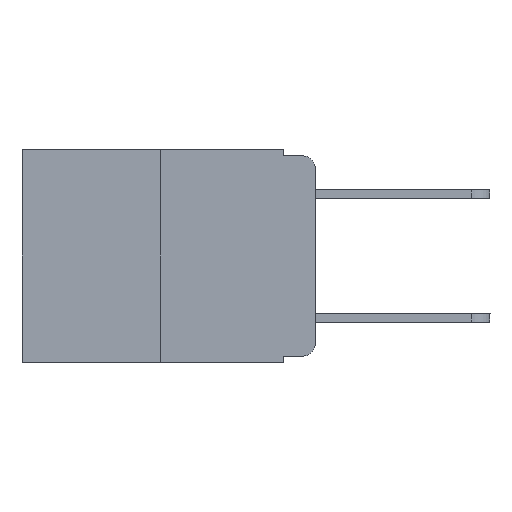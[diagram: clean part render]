
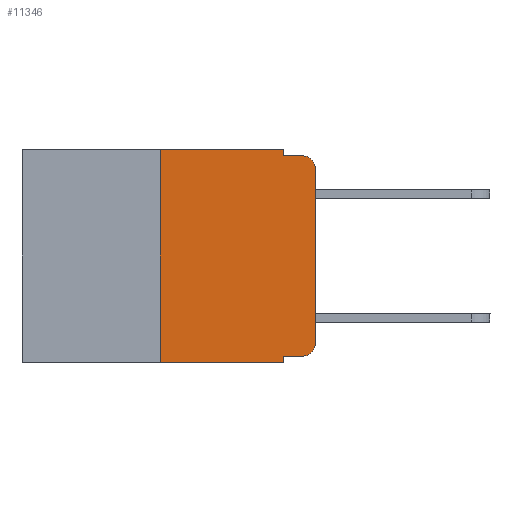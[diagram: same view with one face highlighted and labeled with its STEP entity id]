
A CAD part, left-side view. The second image highlights one B-rep face of the part: STEP entity #11346.
In plain terms, the highlighted planar face has unit normal (-1, 0, 0).
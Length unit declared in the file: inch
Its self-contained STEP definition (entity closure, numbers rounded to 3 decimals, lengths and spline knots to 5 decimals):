
#182 = CARTESIAN_POINT ( 'NONE',  ( 0., 0.473, -0.343 ) ) ;
#188 = ORIENTED_EDGE ( 'NONE', *, *, #4877, .F. ) ;
#247 = EDGE_CURVE ( 'NONE', #12793, #11133, #13879, .T. ) ;
#274 = LINE ( 'NONE', #15302, #7485 ) ;
#284 = VERTEX_POINT ( 'NONE', #14861 ) ;
#427 = EDGE_CURVE ( 'NONE', #15644, #6108, #481, .T. ) ;
#481 = LINE ( 'NONE', #17025, #3374 ) ;
#1415 = LINE ( 'NONE', #182, #1632 ) ;
#1632 = VECTOR ( 'NONE', #8523, 39.37008 ) ;
#1796 = VECTOR ( 'NONE', #3909, 39.37008 ) ;
#1911 = FACE_OUTER_BOUND ( 'NONE', #7385, .T. ) ;
#1937 = LINE ( 'NONE', #13907, #8897 ) ;
#2059 = VECTOR ( 'NONE', #12054, 39.37008 ) ;
#2407 = LINE ( 'NONE', #16637, #6973 ) ;
#2510 = DIRECTION ( 'NONE',  ( 0., 0., -1. ) ) ;
#2595 = CARTESIAN_POINT ( 'NONE',  ( 0., 0.02, -0.01 ) ) ;
#3010 = CARTESIAN_POINT ( 'NONE',  ( 0., 0.02, -0.313 ) ) ;
#3228 = CARTESIAN_POINT ( 'NONE',  ( 0., 0.25, 0. ) ) ;
#3237 = VERTEX_POINT ( 'NONE', #4588 ) ;
#3374 = VECTOR ( 'NONE', #9848, 39.37008 ) ;
#3633 = DIRECTION ( 'NONE',  ( 0., -1., 0. ) ) ;
#3909 = DIRECTION ( 'NONE',  ( 0., 0., -1. ) ) ;
#3939 = EDGE_CURVE ( 'NONE', #3237, #14921, #1937, .T. ) ;
#4208 = LINE ( 'NONE', #10913, #1796 ) ;
#4588 = CARTESIAN_POINT ( 'NONE',  ( 0., 0.25, -0.343 ) ) ;
#4752 = CARTESIAN_POINT ( 'NONE',  ( 0., 0.051, -0.343 ) ) ;
#4877 = EDGE_CURVE ( 'NONE', #14921, #4884, #2407, .T. ) ;
#4884 = VERTEX_POINT ( 'NONE', #15149 ) ;
#5316 = VECTOR ( 'NONE', #3633, 39.37008 ) ;
#5941 = AXIS2_PLACEMENT_3D ( 'NONE', #6714, #6777, #18105 ) ;
#6108 = VERTEX_POINT ( 'NONE', #2595 ) ;
#6363 = CARTESIAN_POINT ( 'NONE',  ( 0., 0.051, -0.333 ) ) ;
#6714 = CARTESIAN_POINT ( 'NONE',  ( 0., 0.02, -0.03 ) ) ;
#6744 = DIRECTION ( 'NONE',  ( 0., -1., 0. ) ) ;
#6777 = DIRECTION ( 'NONE',  ( -1., 0., 0. ) ) ;
#6973 = VECTOR ( 'NONE', #6744, 39.37008 ) ;
#7005 = CIRCLE ( 'NONE', #5941, 0.02 ) ;
#7385 = EDGE_LOOP ( 'NONE', ( #10083, #10742, #11824, #16550, #188, #18148, #14238, #15780, #8867, #13104 ) ) ;
#7485 = VECTOR ( 'NONE', #2510, 39.37008 ) ;
#7997 = EDGE_CURVE ( 'NONE', #4884, #15644, #274, .T. ) ;
#8474 = DIRECTION ( 'NONE',  ( 1., 0., 0. ) ) ;
#8523 = DIRECTION ( 'NONE',  ( 0., -1., 0. ) ) ;
#8645 = CARTESIAN_POINT ( 'NONE',  ( 0., 0.473, 0. ) ) ;
#8788 = EDGE_CURVE ( 'NONE', #284, #16477, #16968, .T. ) ;
#8867 = ORIENTED_EDGE ( 'NONE', *, *, #8788, .T. ) ;
#8897 = VECTOR ( 'NONE', #15712, 39.37008 ) ;
#9082 = AXIS2_PLACEMENT_3D ( 'NONE', #8645, #8474, #14008 ) ;
#9164 = CIRCLE ( 'NONE', #16539, 0.02 ) ;
#9224 = CARTESIAN_POINT ( 'NONE',  ( 0., 0.051, -0.01 ) ) ;
#9396 = EDGE_CURVE ( 'NONE', #284, #13156, #4208, .T. ) ;
#9848 = DIRECTION ( 'NONE',  ( 0., -1., 0. ) ) ;
#10083 = ORIENTED_EDGE ( 'NONE', *, *, #247, .T. ) ;
#10102 = EDGE_CURVE ( 'NONE', #11133, #6108, #7005, .T. ) ;
#10328 = EDGE_CURVE ( 'NONE', #16477, #12793, #9164, .T. ) ;
#10742 = ORIENTED_EDGE ( 'NONE', *, *, #10102, .T. ) ;
#10913 = CARTESIAN_POINT ( 'NONE',  ( 0., 0.051, 0. ) ) ;
#11133 = VERTEX_POINT ( 'NONE', #17987 ) ;
#11346 = ADVANCED_FACE ( 'NONE', ( #1911 ), #17132, .F. ) ;
#11362 = CARTESIAN_POINT ( 'NONE',  ( 0., 0., -0.313 ) ) ;
#11824 = ORIENTED_EDGE ( 'NONE', *, *, #427, .F. ) ;
#12054 = DIRECTION ( 'NONE',  ( 0., 0., 1. ) ) ;
#12774 = EDGE_CURVE ( 'NONE', #3237, #13156, #1415, .T. ) ;
#12793 = VERTEX_POINT ( 'NONE', #11362 ) ;
#13104 = ORIENTED_EDGE ( 'NONE', *, *, #10328, .T. ) ;
#13156 = VERTEX_POINT ( 'NONE', #4752 ) ;
#13879 = LINE ( 'NONE', #14981, #2059 ) ;
#13907 = CARTESIAN_POINT ( 'NONE',  ( 0., 0.25, 0. ) ) ;
#14008 = DIRECTION ( 'NONE',  ( 0., 0., -1. ) ) ;
#14047 = DIRECTION ( 'NONE',  ( -1., 0., 0. ) ) ;
#14238 = ORIENTED_EDGE ( 'NONE', *, *, #12774, .T. ) ;
#14861 = CARTESIAN_POINT ( 'NONE',  ( 0., 0.051, -0.333 ) ) ;
#14921 = VERTEX_POINT ( 'NONE', #3228 ) ;
#14981 = CARTESIAN_POINT ( 'NONE',  ( 0., 0., 0. ) ) ;
#15149 = CARTESIAN_POINT ( 'NONE',  ( 0., 0.051, 0. ) ) ;
#15302 = CARTESIAN_POINT ( 'NONE',  ( 0., 0.051, 0. ) ) ;
#15401 = CARTESIAN_POINT ( 'NONE',  ( 0., 0.02, -0.333 ) ) ;
#15644 = VERTEX_POINT ( 'NONE', #9224 ) ;
#15712 = DIRECTION ( 'NONE',  ( 0., 0., 1. ) ) ;
#15780 = ORIENTED_EDGE ( 'NONE', *, *, #9396, .F. ) ;
#16477 = VERTEX_POINT ( 'NONE', #15401 ) ;
#16539 = AXIS2_PLACEMENT_3D ( 'NONE', #3010, #14047, #17055 ) ;
#16550 = ORIENTED_EDGE ( 'NONE', *, *, #7997, .F. ) ;
#16637 = CARTESIAN_POINT ( 'NONE',  ( 0., 0.473, 0. ) ) ;
#16968 = LINE ( 'NONE', #6363, #5316 ) ;
#17025 = CARTESIAN_POINT ( 'NONE',  ( 0., 0.051, -0.01 ) ) ;
#17055 = DIRECTION ( 'NONE',  ( 0., 0., -1. ) ) ;
#17132 = PLANE ( 'NONE',  #9082 ) ;
#17987 = CARTESIAN_POINT ( 'NONE',  ( 0., 0., -0.03 ) ) ;
#18105 = DIRECTION ( 'NONE',  ( 0., 0., -1. ) ) ;
#18148 = ORIENTED_EDGE ( 'NONE', *, *, #3939, .F. ) ;
